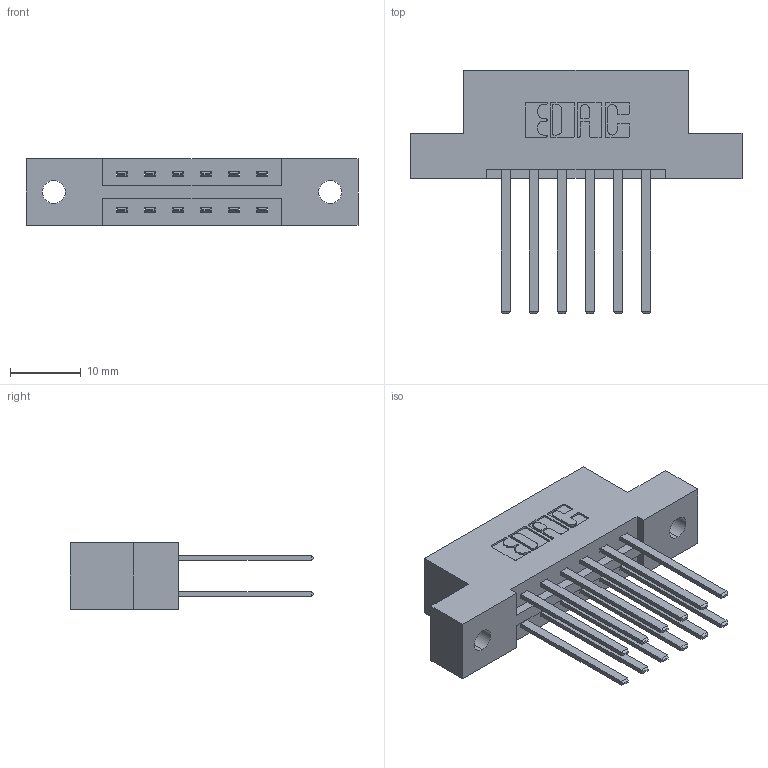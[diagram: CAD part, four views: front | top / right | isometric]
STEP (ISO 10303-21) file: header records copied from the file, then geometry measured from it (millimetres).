
FILE_DESCRIPTION (( 'STEP AP203' ), '1' );
FILE_NAME ('337-012-544-202.STEP', '2018-08-04T04:49:26', ( '' ), ( '' ), 'SwSTEP 2.0', 'SolidWorks 2016', '' );
FILE_SCHEMA (( 'CONFIG_CONTROL_DESIGN' ));
Length unit declared in the file: inch
Products named in the file (3): 337 Part_Flush Mounting Lugs - 0.128 Dia; 345-292-001_345-293-144; 337-012-544-202
Assembly tree (13 placements, depth 2):
  337-012-544-202
    337 Part_Flush Mounting Lugs - 0.128 Dia
    345-292-001_345-293-144  x12
Bounding box: 46.79 x 34.3 x 9.4 mm (x, y, z)
Volume: 4583.1 mm3; surface area: 5108.3 mm2
Topology: 13 solids, 13 shells, 690 faces, 2027 edges, 1334 vertices
Faces by surface type: plane 478, cylinder 212
Entity records: 9127 total; most frequent: CARTESIAN_POINT 1566, ORIENTED_EDGE 1502, DIRECTION 1395, EDGE_CURVE 751, VECTOR 627, LINE 627, VERTEX_POINT 498, AXIS2_PLACEMENT_3D 384
